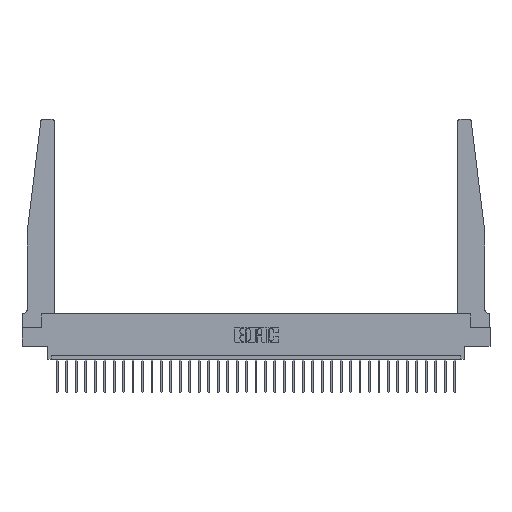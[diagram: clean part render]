
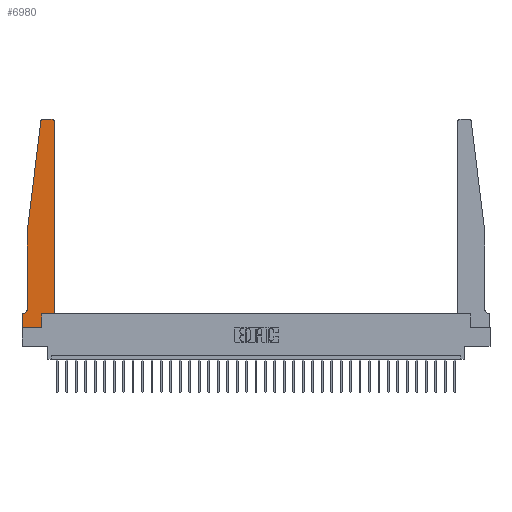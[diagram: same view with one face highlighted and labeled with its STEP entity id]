
A CAD part, top view. The second image highlights one B-rep face of the part: STEP entity #6980.
In plain terms, the highlighted planar face has unit normal (0, 0, 1).
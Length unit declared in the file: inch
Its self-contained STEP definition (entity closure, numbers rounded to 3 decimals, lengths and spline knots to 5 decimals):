
#548 = CARTESIAN_POINT ( 'NONE',  ( 0.24675, 2.72367, 0.37 ) ) ;
#890 = CARTESIAN_POINT ( 'NONE',  ( 0.2605, 0., 0.37 ) ) ;
#1766 = CARTESIAN_POINT ( 'NONE',  ( 0.015, 0.1875, 0.37 ) ) ;
#1976 = ORIENTED_EDGE ( 'NONE', *, *, #3555, .T. ) ;
#2165 = CARTESIAN_POINT ( 'NONE',  ( 0.25, 2.75, 0.37 ) ) ;
#3356 = DIRECTION ( 'NONE',  ( 0., 0., 1. ) ) ;
#3383 = EDGE_CURVE ( 'NONE', #24151, #9988, #7837, .T. ) ;
#3555 = EDGE_CURVE ( 'NONE', #10816, #13374, #17993, .T. ) ;
#3593 = EDGE_CURVE ( 'NONE', #21061, #17720, #31226, .T. ) ;
#3664 = AXIS2_PLACEMENT_3D ( 'NONE', #29159, #9600, #17025 ) ;
#4348 = CARTESIAN_POINT ( 'NONE',  ( 0., 0., 0.37 ) ) ;
#4393 = AXIS2_PLACEMENT_3D ( 'NONE', #12673, #20085, #17503 ) ;
#4861 = CARTESIAN_POINT ( 'NONE',  ( 0., 0.1875, 0.37 ) ) ;
#5609 = EDGE_CURVE ( 'NONE', #15726, #17557, #15948, .T. ) ;
#6087 = ORIENTED_EDGE ( 'NONE', *, *, #3593, .T. ) ;
#6276 = LINE ( 'NONE', #9018, #7660 ) ;
#6980 = ADVANCED_FACE ( 'NONE', ( #25851 ), #29182, .T. ) ;
#7614 = ORIENTED_EDGE ( 'NONE', *, *, #27196, .T. ) ;
#7660 = VECTOR ( 'NONE', #20974, 39.37008 ) ;
#7837 = LINE ( 'NONE', #19341, #15979 ) ;
#8255 = DIRECTION ( 'NONE',  ( -1., 0., 0. ) ) ;
#8410 = EDGE_CURVE ( 'NONE', #17557, #25317, #9666, .T. ) ;
#8530 = CARTESIAN_POINT ( 'NONE',  ( 0.065, 0.2375, 0.37 ) ) ;
#9018 = CARTESIAN_POINT ( 'NONE',  ( 0.425, 0.18, 0.37 ) ) ;
#9332 = CIRCLE ( 'NONE', #3664, 0.03 ) ;
#9441 = ORIENTED_EDGE ( 'NONE', *, *, #15071, .T. ) ;
#9600 = DIRECTION ( 'NONE',  ( 0., 0., 1. ) ) ;
#9666 = LINE ( 'NONE', #26644, #14796 ) ;
#9744 = EDGE_CURVE ( 'NONE', #18532, #26596, #27757, .T. ) ;
#9988 = VERTEX_POINT ( 'NONE', #27408 ) ;
#10110 = CARTESIAN_POINT ( 'NONE',  ( 0.425, 0.18, 0.37 ) ) ;
#10374 = CARTESIAN_POINT ( 'NONE',  ( 0.065, 0.1875, 0.37 ) ) ;
#10479 = ORIENTED_EDGE ( 'NONE', *, *, #20331, .T. ) ;
#10723 = VECTOR ( 'NONE', #8255, 39.37008 ) ;
#10794 = AXIS2_PLACEMENT_3D ( 'NONE', #11140, #12064, #20988 ) ;
#10816 = VERTEX_POINT ( 'NONE', #4861 ) ;
#10894 = CARTESIAN_POINT ( 'NONE',  ( 0., 0., 0.37 ) ) ;
#10933 = ORIENTED_EDGE ( 'NONE', *, *, #8410, .T. ) ;
#11099 = DIRECTION ( 'NONE',  ( 0., 1., 0. ) ) ;
#11140 = CARTESIAN_POINT ( 'NONE',  ( 0., 0.1875, 0.37 ) ) ;
#12064 = DIRECTION ( 'NONE',  ( 0., 0., 1. ) ) ;
#12226 = CARTESIAN_POINT ( 'NONE',  ( 0., 0., 0.37 ) ) ;
#12454 = EDGE_CURVE ( 'NONE', #13374, #24151, #24701, .T. ) ;
#12673 = CARTESIAN_POINT ( 'NONE',  ( 0.015, 0.2375, 0.37 ) ) ;
#13211 = DIRECTION ( 'NONE',  ( 1., 0., 0. ) ) ;
#13374 = VERTEX_POINT ( 'NONE', #12226 ) ;
#14796 = VECTOR ( 'NONE', #24535, 39.37008 ) ;
#15071 = EDGE_CURVE ( 'NONE', #17720, #15726, #9332, .T. ) ;
#15082 = LINE ( 'NONE', #10374, #10723 ) ;
#15327 = CARTESIAN_POINT ( 'NONE',  ( 0.425, 0.18, 0.37 ) ) ;
#15509 = VECTOR ( 'NONE', #16775, 39.37008 ) ;
#15726 = VERTEX_POINT ( 'NONE', #548 ) ;
#15948 = LINE ( 'NONE', #25490, #23486 ) ;
#15979 = VECTOR ( 'NONE', #24191, 39.37008 ) ;
#16528 = CARTESIAN_POINT ( 'NONE',  ( 0.27653, 2.75, 0.37 ) ) ;
#16775 = DIRECTION ( 'NONE',  ( 1., 0., 0. ) ) ;
#17025 = DIRECTION ( 'NONE',  ( 1., 0., 0. ) ) ;
#17287 = CIRCLE ( 'NONE', #18823, 0.03 ) ;
#17503 = DIRECTION ( 'NONE',  ( -1., 0., 0. ) ) ;
#17557 = VERTEX_POINT ( 'NONE', #27560 ) ;
#17720 = VERTEX_POINT ( 'NONE', #16528 ) ;
#17993 = LINE ( 'NONE', #10894, #22686 ) ;
#18323 = CIRCLE ( 'NONE', #4393, 0.05 ) ;
#18445 = VECTOR ( 'NONE', #11099, 39.37008 ) ;
#18516 = CARTESIAN_POINT ( 'NONE',  ( 0.395, 2.75, 0.37 ) ) ;
#18532 = VERTEX_POINT ( 'NONE', #10110 ) ;
#18724 = EDGE_LOOP ( 'NONE', ( #6087, #9441, #31848, #10933, #10479, #18979, #1976, #27557, #21367, #7614, #27649, #21545 ) ) ;
#18823 = AXIS2_PLACEMENT_3D ( 'NONE', #30653, #3356, #13211 ) ;
#18979 = ORIENTED_EDGE ( 'NONE', *, *, #26549, .T. ) ;
#19341 = CARTESIAN_POINT ( 'NONE',  ( 0.2605, 0.18, 0.37 ) ) ;
#20085 = DIRECTION ( 'NONE',  ( 0., 0., -1. ) ) ;
#20117 = EDGE_CURVE ( 'NONE', #26596, #21061, #17287, .T. ) ;
#20331 = EDGE_CURVE ( 'NONE', #25317, #27338, #18323, .T. ) ;
#20743 = DIRECTION ( 'NONE',  ( 0., -1., 0. ) ) ;
#20974 = DIRECTION ( 'NONE',  ( 1., 0., 0. ) ) ;
#20988 = DIRECTION ( 'NONE',  ( 1., 0., 0. ) ) ;
#21061 = VERTEX_POINT ( 'NONE', #18516 ) ;
#21367 = ORIENTED_EDGE ( 'NONE', *, *, #3383, .T. ) ;
#21545 = ORIENTED_EDGE ( 'NONE', *, *, #20117, .T. ) ;
#22686 = VECTOR ( 'NONE', #20743, 39.37008 ) ;
#23204 = DIRECTION ( 'NONE',  ( -0.122, -0.992, 0. ) ) ;
#23486 = VECTOR ( 'NONE', #23204, 39.37008 ) ;
#24151 = VERTEX_POINT ( 'NONE', #890 ) ;
#24191 = DIRECTION ( 'NONE',  ( 0., 1., 0. ) ) ;
#24535 = DIRECTION ( 'NONE',  ( 0., -1., 0. ) ) ;
#24701 = LINE ( 'NONE', #4348, #15509 ) ;
#25317 = VERTEX_POINT ( 'NONE', #8530 ) ;
#25490 = CARTESIAN_POINT ( 'NONE',  ( 0.065, 1.25, 0.37 ) ) ;
#25851 = FACE_OUTER_BOUND ( 'NONE', #18724, .T. ) ;
#26549 = EDGE_CURVE ( 'NONE', #27338, #10816, #15082, .T. ) ;
#26596 = VERTEX_POINT ( 'NONE', #30085 ) ;
#26644 = CARTESIAN_POINT ( 'NONE',  ( 0.065, 1.25, 0.37 ) ) ;
#27196 = EDGE_CURVE ( 'NONE', #9988, #18532, #6276, .T. ) ;
#27338 = VERTEX_POINT ( 'NONE', #1766 ) ;
#27408 = CARTESIAN_POINT ( 'NONE',  ( 0.2605, 0.18, 0.37 ) ) ;
#27557 = ORIENTED_EDGE ( 'NONE', *, *, #12454, .T. ) ;
#27560 = CARTESIAN_POINT ( 'NONE',  ( 0.065, 1.25, 0.37 ) ) ;
#27649 = ORIENTED_EDGE ( 'NONE', *, *, #9744, .T. ) ;
#27757 = LINE ( 'NONE', #15327, #18445 ) ;
#29132 = DIRECTION ( 'NONE',  ( -1., 0., 0. ) ) ;
#29159 = CARTESIAN_POINT ( 'NONE',  ( 0.27653, 2.72, 0.37 ) ) ;
#29182 = PLANE ( 'NONE',  #10794 ) ;
#30085 = CARTESIAN_POINT ( 'NONE',  ( 0.425, 2.72, 0.37 ) ) ;
#30409 = VECTOR ( 'NONE', #29132, 39.37008 ) ;
#30653 = CARTESIAN_POINT ( 'NONE',  ( 0.395, 2.72, 0.37 ) ) ;
#31226 = LINE ( 'NONE', #2165, #30409 ) ;
#31848 = ORIENTED_EDGE ( 'NONE', *, *, #5609, .T. ) ;
